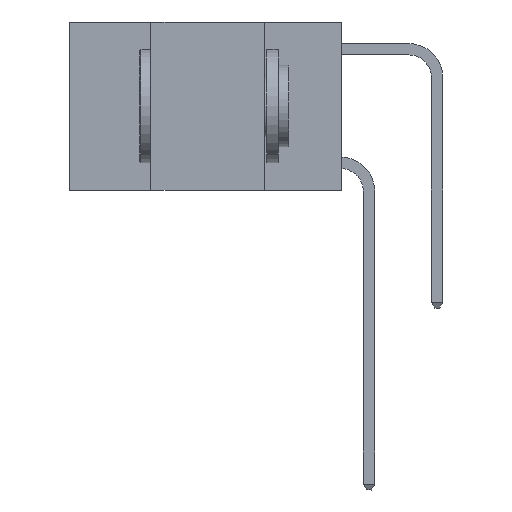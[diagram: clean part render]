
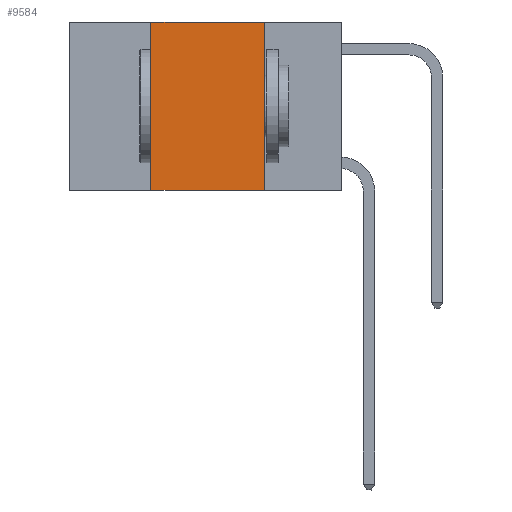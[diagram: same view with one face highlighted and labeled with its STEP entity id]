
A CAD part, left-side view. The second image highlights one B-rep face of the part: STEP entity #9584.
In plain terms, the highlighted planar face has unit normal (-1, 0, 0).
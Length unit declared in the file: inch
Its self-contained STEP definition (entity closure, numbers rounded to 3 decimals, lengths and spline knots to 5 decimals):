
#371 = LINE ( 'NONE', #8894, #13042 ) ;
#840 = LINE ( 'NONE', #11633, #5372 ) ;
#1254 = VERTEX_POINT ( 'NONE', #2590 ) ;
#1450 = VERTEX_POINT ( 'NONE', #13709 ) ;
#1575 = EDGE_CURVE ( 'NONE', #4437, #2839, #10221, .T. ) ;
#1821 = VECTOR ( 'NONE', #2003, 39.37008 ) ;
#2003 = DIRECTION ( 'NONE',  ( 0., -1., 0. ) ) ;
#2322 = EDGE_LOOP ( 'NONE', ( #6215, #9297, #10035, #13016 ) ) ;
#2590 = CARTESIAN_POINT ( 'NONE',  ( 0., 0.17, -0.37 ) ) ;
#2839 = VERTEX_POINT ( 'NONE', #6740 ) ;
#3074 = CARTESIAN_POINT ( 'NONE',  ( 0., 0.6, -0.37 ) ) ;
#3599 = DIRECTION ( 'NONE',  ( 0., -1., 0. ) ) ;
#3730 = EDGE_CURVE ( 'NONE', #2839, #1450, #371, .T. ) ;
#3843 = CARTESIAN_POINT ( 'NONE',  ( 0., 0.42, 0. ) ) ;
#4021 = PLANE ( 'NONE',  #8943 ) ;
#4167 = DIRECTION ( 'NONE',  ( 1., 0., 0. ) ) ;
#4222 = CARTESIAN_POINT ( 'NONE',  ( 0., 0.6, 0. ) ) ;
#4437 = VERTEX_POINT ( 'NONE', #10455 ) ;
#5069 = DIRECTION ( 'NONE',  ( 0., 0., -1. ) ) ;
#5372 = VECTOR ( 'NONE', #10448, 39.37008 ) ;
#6215 = ORIENTED_EDGE ( 'NONE', *, *, #8731, .F. ) ;
#6740 = CARTESIAN_POINT ( 'NONE',  ( 0., 0.42, 0. ) ) ;
#6978 = VECTOR ( 'NONE', #9129, 39.37008 ) ;
#8731 = EDGE_CURVE ( 'NONE', #1450, #1254, #840, .T. ) ;
#8894 = CARTESIAN_POINT ( 'NONE',  ( 0., 0.6, 0. ) ) ;
#8943 = AXIS2_PLACEMENT_3D ( 'NONE', #4222, #4167, #5069 ) ;
#9129 = DIRECTION ( 'NONE',  ( 0., 0., 1. ) ) ;
#9297 = ORIENTED_EDGE ( 'NONE', *, *, #3730, .F. ) ;
#9584 = ADVANCED_FACE ( 'NONE', ( #10398 ), #4021, .F. ) ;
#10035 = ORIENTED_EDGE ( 'NONE', *, *, #1575, .F. ) ;
#10221 = LINE ( 'NONE', #3843, #6978 ) ;
#10398 = FACE_OUTER_BOUND ( 'NONE', #2322, .T. ) ;
#10448 = DIRECTION ( 'NONE',  ( 0., 0., -1. ) ) ;
#10455 = CARTESIAN_POINT ( 'NONE',  ( 0., 0.42, -0.37 ) ) ;
#11633 = CARTESIAN_POINT ( 'NONE',  ( 0., 0.17, 0. ) ) ;
#12453 = EDGE_CURVE ( 'NONE', #4437, #1254, #12680, .T. ) ;
#12680 = LINE ( 'NONE', #3074, #1821 ) ;
#13016 = ORIENTED_EDGE ( 'NONE', *, *, #12453, .T. ) ;
#13042 = VECTOR ( 'NONE', #3599, 39.37008 ) ;
#13709 = CARTESIAN_POINT ( 'NONE',  ( 0., 0.17, 0. ) ) ;
